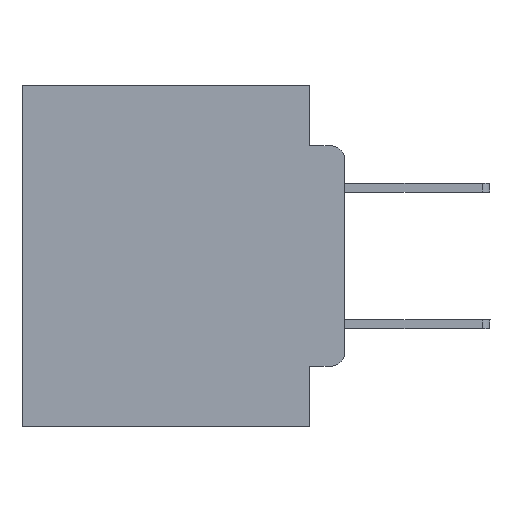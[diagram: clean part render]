
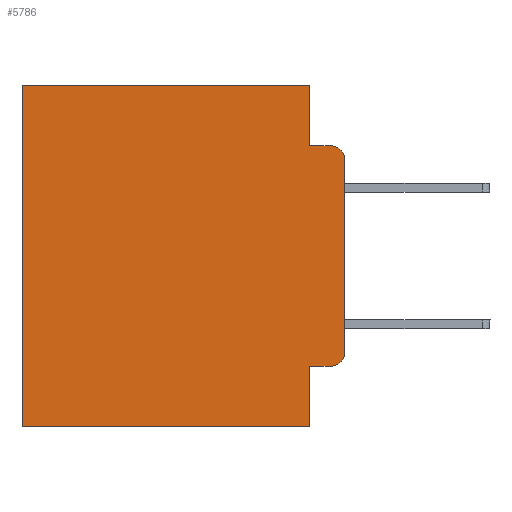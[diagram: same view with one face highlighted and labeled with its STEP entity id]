
A CAD part, left-side view. The second image highlights one B-rep face of the part: STEP entity #5786.
In plain terms, the highlighted planar face has unit normal (-1, 0, 0).
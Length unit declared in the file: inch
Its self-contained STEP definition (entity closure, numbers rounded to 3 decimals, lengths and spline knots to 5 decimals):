
#690 = CARTESIAN_POINT ( 'NONE',  ( 0.298, 0., 0. ) ) ;
#1453 = DIRECTION ( 'NONE',  ( 0., 1., 0. ) ) ;
#1845 = VERTEX_POINT ( 'NONE', #2702 ) ;
#1998 = LINE ( 'NONE', #2261, #25886 ) ;
#2261 = CARTESIAN_POINT ( 'NONE',  ( 0.298, 0.473, 0. ) ) ;
#2557 = VECTOR ( 'NONE', #26500, 39.37008 ) ;
#2702 = CARTESIAN_POINT ( 'NONE',  ( 0.298, 0., -0.1085 ) ) ;
#3262 = CARTESIAN_POINT ( 'NONE',  ( 0.298, 0.02, -0.1085 ) ) ;
#3630 = DIRECTION ( 'NONE',  ( -1., 0., 0. ) ) ;
#3637 = EDGE_CURVE ( 'NONE', #17564, #6093, #25011, .T. ) ;
#3698 = CARTESIAN_POINT ( 'NONE',  ( 0.298, 0., 0. ) ) ;
#4000 = CIRCLE ( 'NONE', #17385, 0.02 ) ;
#4563 = VERTEX_POINT ( 'NONE', #9167 ) ;
#4577 = FACE_OUTER_BOUND ( 'NONE', #10746, .T. ) ;
#4799 = EDGE_CURVE ( 'NONE', #6093, #19359, #4000, .T. ) ;
#5086 = EDGE_CURVE ( 'NONE', #15091, #19815, #5645, .T. ) ;
#5227 = LINE ( 'NONE', #9757, #14427 ) ;
#5627 = LINE ( 'NONE', #23915, #21687 ) ;
#5645 = LINE ( 'NONE', #19739, #15790 ) ;
#5786 = ADVANCED_FACE ( 'NONE', ( #4577 ), #25850, .F. ) ;
#5965 = CARTESIAN_POINT ( 'NONE',  ( 0.298, 0.051, -0.4115 ) ) ;
#6093 = VERTEX_POINT ( 'NONE', #21241 ) ;
#6358 = ORIENTED_EDGE ( 'NONE', *, *, #22632, .T. ) ;
#7231 = EDGE_CURVE ( 'NONE', #16381, #21092, #5227, .T. ) ;
#8086 = LINE ( 'NONE', #10007, #2557 ) ;
#8262 = ORIENTED_EDGE ( 'NONE', *, *, #4799, .T. ) ;
#8710 = ORIENTED_EDGE ( 'NONE', *, *, #5086, .F. ) ;
#8748 = VECTOR ( 'NONE', #13115, 39.37008 ) ;
#9136 = ORIENTED_EDGE ( 'NONE', *, *, #24766, .T. ) ;
#9167 = CARTESIAN_POINT ( 'NONE',  ( 0.298, 0.051, 0. ) ) ;
#9350 = DIRECTION ( 'NONE',  ( 0., 0., -1. ) ) ;
#9472 = CARTESIAN_POINT ( 'NONE',  ( 0.298, 0., -0.3915 ) ) ;
#9649 = ORIENTED_EDGE ( 'NONE', *, *, #7231, .F. ) ;
#9757 = CARTESIAN_POINT ( 'NONE',  ( 0.298, 0.051, -0.0885 ) ) ;
#10007 = CARTESIAN_POINT ( 'NONE',  ( 0.298, 0.051, 0. ) ) ;
#10746 = EDGE_LOOP ( 'NONE', ( #12230, #6358, #9649, #12288, #23716, #9136, #8710, #17137, #14792, #8262 ) ) ;
#11678 = DIRECTION ( 'NONE',  ( 0., 0., -1. ) ) ;
#12230 = ORIENTED_EDGE ( 'NONE', *, *, #20083, .F. ) ;
#12288 = ORIENTED_EDGE ( 'NONE', *, *, #23851, .F. ) ;
#12665 = DIRECTION ( 'NONE',  ( 0., 0., -1. ) ) ;
#13115 = DIRECTION ( 'NONE',  ( 0., 0., -1. ) ) ;
#13464 = CARTESIAN_POINT ( 'NONE',  ( 0.298, 0.051, -0.0885 ) ) ;
#14123 = DIRECTION ( 'NONE',  ( -1., 0., 0. ) ) ;
#14130 = DIRECTION ( 'NONE',  ( 0., -1., 0. ) ) ;
#14422 = VECTOR ( 'NONE', #1453, 39.37008 ) ;
#14427 = VECTOR ( 'NONE', #18059, 39.37008 ) ;
#14538 = VECTOR ( 'NONE', #14130, 39.37008 ) ;
#14792 = ORIENTED_EDGE ( 'NONE', *, *, #3637, .T. ) ;
#15091 = VERTEX_POINT ( 'NONE', #21184 ) ;
#15790 = VECTOR ( 'NONE', #25974, 39.37008 ) ;
#16381 = VERTEX_POINT ( 'NONE', #13464 ) ;
#16710 = CARTESIAN_POINT ( 'NONE',  ( 0.298, 0.02, -0.0885 ) ) ;
#17137 = ORIENTED_EDGE ( 'NONE', *, *, #20282, .F. ) ;
#17385 = AXIS2_PLACEMENT_3D ( 'NONE', #20605, #14123, #27008 ) ;
#17564 = VERTEX_POINT ( 'NONE', #5965 ) ;
#17770 = DIRECTION ( 'NONE',  ( 1., 0., 0. ) ) ;
#18059 = DIRECTION ( 'NONE',  ( 0., -1., 0. ) ) ;
#18697 = CARTESIAN_POINT ( 'NONE',  ( 0.298, 0.473, 0. ) ) ;
#18927 = AXIS2_PLACEMENT_3D ( 'NONE', #3262, #3630, #11678 ) ;
#19359 = VERTEX_POINT ( 'NONE', #9472 ) ;
#19430 = DIRECTION ( 'NONE',  ( 0., 0., -1. ) ) ;
#19727 = CIRCLE ( 'NONE', #18927, 0.02 ) ;
#19739 = CARTESIAN_POINT ( 'NONE',  ( 0.298, 0., -0.5 ) ) ;
#19761 = VERTEX_POINT ( 'NONE', #18697 ) ;
#19815 = VERTEX_POINT ( 'NONE', #20563 ) ;
#20083 = EDGE_CURVE ( 'NONE', #1845, #19359, #23200, .T. ) ;
#20282 = EDGE_CURVE ( 'NONE', #17564, #15091, #8086, .T. ) ;
#20563 = CARTESIAN_POINT ( 'NONE',  ( 0.298, 0.473, -0.5 ) ) ;
#20605 = CARTESIAN_POINT ( 'NONE',  ( 0.298, 0.02, -0.3915 ) ) ;
#21092 = VERTEX_POINT ( 'NONE', #16710 ) ;
#21184 = CARTESIAN_POINT ( 'NONE',  ( 0.298, 0.051, -0.5 ) ) ;
#21241 = CARTESIAN_POINT ( 'NONE',  ( 0.298, 0.02, -0.4115 ) ) ;
#21364 = CARTESIAN_POINT ( 'NONE',  ( 0.298, 0., 0. ) ) ;
#21687 = VECTOR ( 'NONE', #9350, 39.37008 ) ;
#22632 = EDGE_CURVE ( 'NONE', #1845, #21092, #19727, .T. ) ;
#23200 = LINE ( 'NONE', #21364, #8748 ) ;
#23716 = ORIENTED_EDGE ( 'NONE', *, *, #25179, .T. ) ;
#23851 = EDGE_CURVE ( 'NONE', #4563, #16381, #5627, .T. ) ;
#23915 = CARTESIAN_POINT ( 'NONE',  ( 0.298, 0.051, 0. ) ) ;
#24457 = AXIS2_PLACEMENT_3D ( 'NONE', #690, #17770, #19430 ) ;
#24766 = EDGE_CURVE ( 'NONE', #19761, #19815, #1998, .T. ) ;
#25011 = LINE ( 'NONE', #26667, #14538 ) ;
#25179 = EDGE_CURVE ( 'NONE', #4563, #19761, #25550, .T. ) ;
#25550 = LINE ( 'NONE', #3698, #14422 ) ;
#25850 = PLANE ( 'NONE',  #24457 ) ;
#25886 = VECTOR ( 'NONE', #12665, 39.37008 ) ;
#25974 = DIRECTION ( 'NONE',  ( 0., 1., 0. ) ) ;
#26500 = DIRECTION ( 'NONE',  ( 0., 0., -1. ) ) ;
#26667 = CARTESIAN_POINT ( 'NONE',  ( 0.298, 0.051, -0.4115 ) ) ;
#27008 = DIRECTION ( 'NONE',  ( 0., 0., -1. ) ) ;
